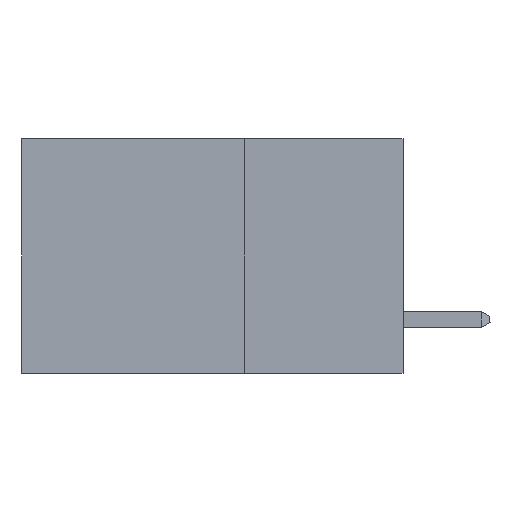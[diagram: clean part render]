
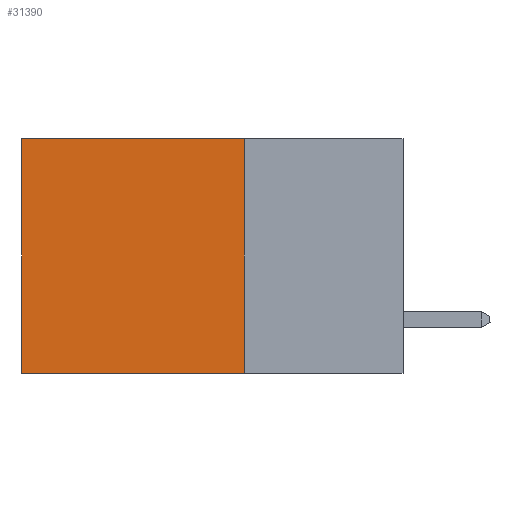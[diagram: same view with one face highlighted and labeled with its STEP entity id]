
A CAD part, left-side view. The second image highlights one B-rep face of the part: STEP entity #31390.
In plain terms, the highlighted planar face has unit normal (-1, 0, 0).
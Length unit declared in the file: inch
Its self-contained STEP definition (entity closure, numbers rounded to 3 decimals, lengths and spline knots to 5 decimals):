
#189 = FACE_OUTER_BOUND ( 'NONE', #23758, .T. ) ;
#348 = ORIENTED_EDGE ( 'NONE', *, *, #40211, .F. ) ;
#1211 = ORIENTED_EDGE ( 'NONE', *, *, #4875, .T. ) ;
#1262 = DIRECTION ( 'NONE',  ( 0., 1., 0. ) ) ;
#3489 = VERTEX_POINT ( 'NONE', #10416 ) ;
#4251 = LINE ( 'NONE', #37226, #20804 ) ;
#4875 = EDGE_CURVE ( 'NONE', #27161, #3489, #5343, .T. ) ;
#5343 = LINE ( 'NONE', #37428, #13110 ) ;
#6310 = VERTEX_POINT ( 'NONE', #32328 ) ;
#7224 = DIRECTION ( 'NONE',  ( 0., 0., -1. ) ) ;
#10362 = DIRECTION ( 'NONE',  ( 1., 0., 0. ) ) ;
#10416 = CARTESIAN_POINT ( 'NONE',  ( 0.2875, 0.6, 0. ) ) ;
#12060 = VECTOR ( 'NONE', #7224, 39.37008 ) ;
#13110 = VECTOR ( 'NONE', #1262, 39.37008 ) ;
#13115 = LINE ( 'NONE', #17088, #12060 ) ;
#17088 = CARTESIAN_POINT ( 'NONE',  ( 0.2875, 0.6, 0. ) ) ;
#17673 = VERTEX_POINT ( 'NONE', #35869 ) ;
#17728 = VECTOR ( 'NONE', #32762, 39.37008 ) ;
#20150 = EDGE_CURVE ( 'NONE', #3489, #6310, #13115, .T. ) ;
#20804 = VECTOR ( 'NONE', #27319, 39.37008 ) ;
#22164 = CARTESIAN_POINT ( 'NONE',  ( 0.2875, 0.25, 0. ) ) ;
#23162 = ORIENTED_EDGE ( 'NONE', *, *, #32171, .F. ) ;
#23758 = EDGE_LOOP ( 'NONE', ( #30821, #348, #23162, #1211 ) ) ;
#27161 = VERTEX_POINT ( 'NONE', #22164 ) ;
#27319 = DIRECTION ( 'NONE',  ( 0., 0., -1. ) ) ;
#29438 = CARTESIAN_POINT ( 'NONE',  ( 0.2875, 0.25, -0.37 ) ) ;
#30118 = CARTESIAN_POINT ( 'NONE',  ( 0.2875, 0.25, 0. ) ) ;
#30821 = ORIENTED_EDGE ( 'NONE', *, *, #20150, .T. ) ;
#31390 = ADVANCED_FACE ( 'NONE', ( #189 ), #33300, .F. ) ;
#32171 = EDGE_CURVE ( 'NONE', #27161, #17673, #4251, .T. ) ;
#32328 = CARTESIAN_POINT ( 'NONE',  ( 0.2875, 0.6, -0.37 ) ) ;
#32762 = DIRECTION ( 'NONE',  ( 0., 1., 0. ) ) ;
#33300 = PLANE ( 'NONE',  #35858 ) ;
#33428 = DIRECTION ( 'NONE',  ( 0., 0., -1. ) ) ;
#35184 = LINE ( 'NONE', #29438, #17728 ) ;
#35858 = AXIS2_PLACEMENT_3D ( 'NONE', #30118, #10362, #33428 ) ;
#35869 = CARTESIAN_POINT ( 'NONE',  ( 0.2875, 0.25, -0.37 ) ) ;
#37226 = CARTESIAN_POINT ( 'NONE',  ( 0.2875, 0.25, 0. ) ) ;
#37428 = CARTESIAN_POINT ( 'NONE',  ( 0.2875, 0.25, 0. ) ) ;
#40211 = EDGE_CURVE ( 'NONE', #17673, #6310, #35184, .T. ) ;
